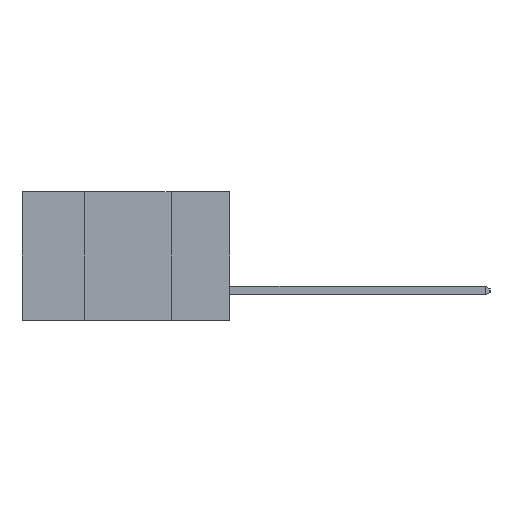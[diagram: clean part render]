
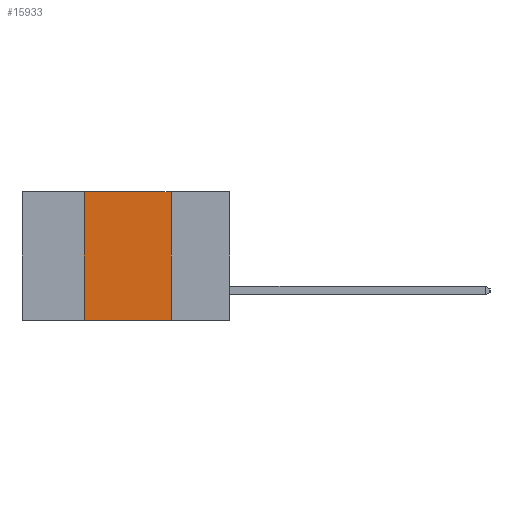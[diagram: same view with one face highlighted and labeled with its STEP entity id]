
A CAD part, left-side view. The second image highlights one B-rep face of the part: STEP entity #15933.
In plain terms, the highlighted planar face has unit normal (-1, 0, 0).
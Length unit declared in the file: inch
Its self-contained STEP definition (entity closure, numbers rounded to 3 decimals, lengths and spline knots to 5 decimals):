
#473 = VECTOR ( 'NONE', #3615, 39.37008 ) ;
#578 = VERTEX_POINT ( 'NONE', #15194 ) ;
#591 = CARTESIAN_POINT ( 'NONE',  ( 0., 0.6, -0.37 ) ) ;
#2021 = EDGE_LOOP ( 'NONE', ( #10920, #13017, #16571, #15894 ) ) ;
#2148 = CARTESIAN_POINT ( 'NONE',  ( 0., 0.17, 0. ) ) ;
#2597 = DIRECTION ( 'NONE',  ( 0., -1., 0. ) ) ;
#3615 = DIRECTION ( 'NONE',  ( 0., 0., -1. ) ) ;
#3782 = EDGE_CURVE ( 'NONE', #6259, #10718, #10777, .T. ) ;
#4202 = PLANE ( 'NONE',  #14916 ) ;
#4598 = CARTESIAN_POINT ( 'NONE',  ( 0., 0.42, 0. ) ) ;
#4874 = VERTEX_POINT ( 'NONE', #17917 ) ;
#5664 = DIRECTION ( 'NONE',  ( 1., 0., 0. ) ) ;
#5983 = VECTOR ( 'NONE', #2597, 39.37008 ) ;
#6053 = LINE ( 'NONE', #10763, #16306 ) ;
#6259 = VERTEX_POINT ( 'NONE', #14357 ) ;
#6339 = EDGE_CURVE ( 'NONE', #10718, #4874, #6053, .T. ) ;
#6445 = LINE ( 'NONE', #591, #5983 ) ;
#8603 = EDGE_CURVE ( 'NONE', #6259, #578, #6445, .T. ) ;
#10718 = VERTEX_POINT ( 'NONE', #4598 ) ;
#10763 = CARTESIAN_POINT ( 'NONE',  ( 0., 0.6, 0. ) ) ;
#10777 = LINE ( 'NONE', #10845, #17576 ) ;
#10845 = CARTESIAN_POINT ( 'NONE',  ( 0., 0.42, 0. ) ) ;
#10861 = DIRECTION ( 'NONE',  ( 0., 0., 1. ) ) ;
#10920 = ORIENTED_EDGE ( 'NONE', *, *, #14514, .F. ) ;
#11994 = LINE ( 'NONE', #2148, #473 ) ;
#12692 = CARTESIAN_POINT ( 'NONE',  ( 0., 0.6, 0. ) ) ;
#12842 = FACE_OUTER_BOUND ( 'NONE', #2021, .T. ) ;
#13017 = ORIENTED_EDGE ( 'NONE', *, *, #6339, .F. ) ;
#14357 = CARTESIAN_POINT ( 'NONE',  ( 0., 0.42, -0.37 ) ) ;
#14514 = EDGE_CURVE ( 'NONE', #4874, #578, #11994, .T. ) ;
#14873 = DIRECTION ( 'NONE',  ( 0., -1., 0. ) ) ;
#14916 = AXIS2_PLACEMENT_3D ( 'NONE', #12692, #5664, #15428 ) ;
#15194 = CARTESIAN_POINT ( 'NONE',  ( 0., 0.17, -0.37 ) ) ;
#15428 = DIRECTION ( 'NONE',  ( 0., 0., -1. ) ) ;
#15894 = ORIENTED_EDGE ( 'NONE', *, *, #8603, .T. ) ;
#15933 = ADVANCED_FACE ( 'NONE', ( #12842 ), #4202, .F. ) ;
#16306 = VECTOR ( 'NONE', #14873, 39.37008 ) ;
#16571 = ORIENTED_EDGE ( 'NONE', *, *, #3782, .F. ) ;
#17576 = VECTOR ( 'NONE', #10861, 39.37008 ) ;
#17917 = CARTESIAN_POINT ( 'NONE',  ( 0., 0.17, 0. ) ) ;
